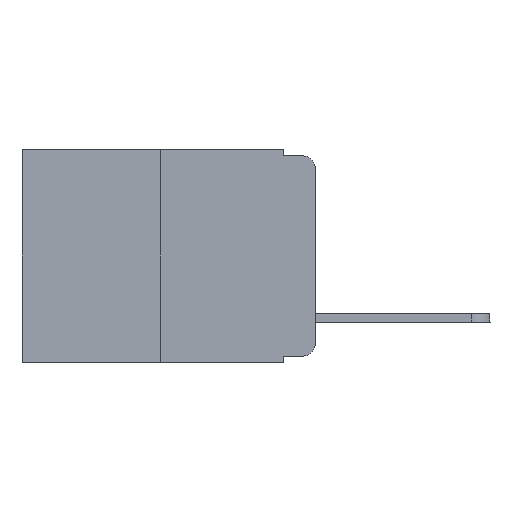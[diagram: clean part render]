
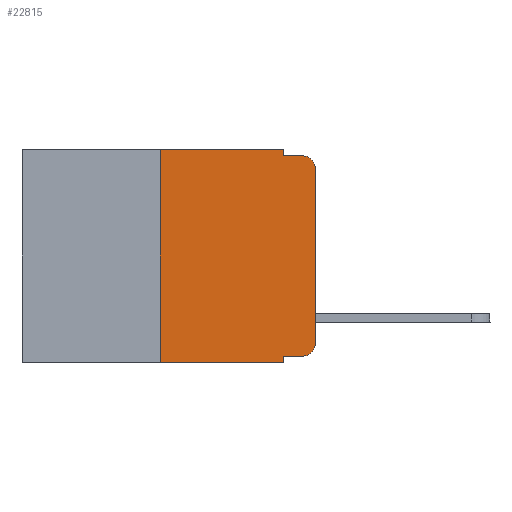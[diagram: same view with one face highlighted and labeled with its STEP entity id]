
A CAD part, left-side view. The second image highlights one B-rep face of the part: STEP entity #22815.
In plain terms, the highlighted planar face has unit normal (-1, 0, 0).
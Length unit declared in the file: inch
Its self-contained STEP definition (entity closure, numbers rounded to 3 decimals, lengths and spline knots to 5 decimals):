
#194 = VERTEX_POINT ( 'NONE', #18640 ) ;
#509 = AXIS2_PLACEMENT_3D ( 'NONE', #10040, #17757, #15505 ) ;
#854 = LINE ( 'NONE', #21071, #17240 ) ;
#1077 = VERTEX_POINT ( 'NONE', #19638 ) ;
#1090 = ORIENTED_EDGE ( 'NONE', *, *, #5804, .F. ) ;
#1209 = VERTEX_POINT ( 'NONE', #13346 ) ;
#1763 = VERTEX_POINT ( 'NONE', #2356 ) ;
#2220 = DIRECTION ( 'NONE',  ( 0., 0., 1. ) ) ;
#2356 = CARTESIAN_POINT ( 'NONE',  ( 0., 0.051, -0.01 ) ) ;
#3010 = VECTOR ( 'NONE', #23158, 39.37008 ) ;
#3176 = VERTEX_POINT ( 'NONE', #6206 ) ;
#3215 = CARTESIAN_POINT ( 'NONE',  ( 0., 0.051, -0.01 ) ) ;
#4160 = CIRCLE ( 'NONE', #19452, 0.02 ) ;
#4940 = VECTOR ( 'NONE', #9705, 39.37008 ) ;
#5382 = VERTEX_POINT ( 'NONE', #6452 ) ;
#5804 = EDGE_CURVE ( 'NONE', #1077, #10270, #8933, .T. ) ;
#5820 = LINE ( 'NONE', #3215, #4940 ) ;
#6116 = ORIENTED_EDGE ( 'NONE', *, *, #10657, .T. ) ;
#6206 = CARTESIAN_POINT ( 'NONE',  ( 0., 0., -0.03 ) ) ;
#6226 = CARTESIAN_POINT ( 'NONE',  ( 0., 0.02, -0.03 ) ) ;
#6452 = CARTESIAN_POINT ( 'NONE',  ( 0., 0.25, -0.343 ) ) ;
#6763 = ORIENTED_EDGE ( 'NONE', *, *, #11725, .T. ) ;
#6996 = ORIENTED_EDGE ( 'NONE', *, *, #19498, .F. ) ;
#7298 = CARTESIAN_POINT ( 'NONE',  ( 0., 0.051, 0. ) ) ;
#7810 = DIRECTION ( 'NONE',  ( 0., 0., -1. ) ) ;
#8051 = CARTESIAN_POINT ( 'NONE',  ( 0., 0.473, 0. ) ) ;
#8629 = ORIENTED_EDGE ( 'NONE', *, *, #8734, .T. ) ;
#8734 = EDGE_CURVE ( 'NONE', #194, #11779, #18633, .T. ) ;
#8880 = LINE ( 'NONE', #19145, #15117 ) ;
#8933 = LINE ( 'NONE', #7298, #20874 ) ;
#9314 = CARTESIAN_POINT ( 'NONE',  ( 0., 0., -0.313 ) ) ;
#9377 = ORIENTED_EDGE ( 'NONE', *, *, #12664, .T. ) ;
#9502 = CARTESIAN_POINT ( 'NONE',  ( 0., 0., 0. ) ) ;
#9517 = LINE ( 'NONE', #13839, #16633 ) ;
#9705 = DIRECTION ( 'NONE',  ( 0., -1., 0. ) ) ;
#9771 = CARTESIAN_POINT ( 'NONE',  ( 0., 0.051, -0.333 ) ) ;
#10040 = CARTESIAN_POINT ( 'NONE',  ( 0., 0.02, -0.313 ) ) ;
#10270 = VERTEX_POINT ( 'NONE', #10436 ) ;
#10436 = CARTESIAN_POINT ( 'NONE',  ( 0., 0.051, -0.343 ) ) ;
#10657 = EDGE_CURVE ( 'NONE', #1077, #194, #13467, .T. ) ;
#10731 = ORIENTED_EDGE ( 'NONE', *, *, #11717, .F. ) ;
#11422 = ORIENTED_EDGE ( 'NONE', *, *, #20151, .F. ) ;
#11717 = EDGE_CURVE ( 'NONE', #20678, #1763, #854, .T. ) ;
#11722 = DIRECTION ( 'NONE',  ( 0., 0., -1. ) ) ;
#11725 = EDGE_CURVE ( 'NONE', #11779, #3176, #18440, .T. ) ;
#11779 = VERTEX_POINT ( 'NONE', #9314 ) ;
#12202 = VECTOR ( 'NONE', #2220, 39.37008 ) ;
#12288 = ORIENTED_EDGE ( 'NONE', *, *, #24498, .T. ) ;
#12664 = EDGE_CURVE ( 'NONE', #5382, #10270, #9517, .T. ) ;
#13051 = ORIENTED_EDGE ( 'NONE', *, *, #19411, .F. ) ;
#13346 = CARTESIAN_POINT ( 'NONE',  ( 0., 0.02, -0.01 ) ) ;
#13467 = LINE ( 'NONE', #9771, #3010 ) ;
#13555 = DIRECTION ( 'NONE',  ( 1., 0., 0. ) ) ;
#13806 = PLANE ( 'NONE',  #21669 ) ;
#13839 = CARTESIAN_POINT ( 'NONE',  ( 0., 0.473, -0.343 ) ) ;
#14164 = VECTOR ( 'NONE', #20880, 39.37008 ) ;
#15117 = VECTOR ( 'NONE', #19065, 39.37008 ) ;
#15505 = DIRECTION ( 'NONE',  ( 0., 0., -1. ) ) ;
#15634 = DIRECTION ( 'NONE',  ( 0., 0., -1. ) ) ;
#15910 = DIRECTION ( 'NONE',  ( 0., -1., 0. ) ) ;
#16633 = VECTOR ( 'NONE', #15910, 39.37008 ) ;
#16689 = EDGE_LOOP ( 'NONE', ( #6763, #12288, #13051, #10731, #6996, #11422, #9377, #1090, #6116, #8629 ) ) ;
#17017 = CARTESIAN_POINT ( 'NONE',  ( 0., 0.473, 0. ) ) ;
#17240 = VECTOR ( 'NONE', #7810, 39.37008 ) ;
#17757 = DIRECTION ( 'NONE',  ( -1., 0., 0. ) ) ;
#18440 = LINE ( 'NONE', #9502, #12202 ) ;
#18633 = CIRCLE ( 'NONE', #509, 0.02 ) ;
#18640 = CARTESIAN_POINT ( 'NONE',  ( 0., 0.02, -0.333 ) ) ;
#18899 = LINE ( 'NONE', #17017, #14164 ) ;
#19065 = DIRECTION ( 'NONE',  ( 0., 0., 1. ) ) ;
#19145 = CARTESIAN_POINT ( 'NONE',  ( 0., 0.25, 0. ) ) ;
#19411 = EDGE_CURVE ( 'NONE', #1763, #1209, #5820, .T. ) ;
#19452 = AXIS2_PLACEMENT_3D ( 'NONE', #6226, #23375, #15634 ) ;
#19498 = EDGE_CURVE ( 'NONE', #21715, #20678, #18899, .T. ) ;
#19638 = CARTESIAN_POINT ( 'NONE',  ( 0., 0.051, -0.333 ) ) ;
#20151 = EDGE_CURVE ( 'NONE', #5382, #21715, #8880, .T. ) ;
#20460 = DIRECTION ( 'NONE',  ( 0., 0., -1. ) ) ;
#20657 = CARTESIAN_POINT ( 'NONE',  ( 0., 0.051, 0. ) ) ;
#20678 = VERTEX_POINT ( 'NONE', #20657 ) ;
#20874 = VECTOR ( 'NONE', #20460, 39.37008 ) ;
#20880 = DIRECTION ( 'NONE',  ( 0., -1., 0. ) ) ;
#21071 = CARTESIAN_POINT ( 'NONE',  ( 0., 0.051, 0. ) ) ;
#21669 = AXIS2_PLACEMENT_3D ( 'NONE', #8051, #13555, #11722 ) ;
#21715 = VERTEX_POINT ( 'NONE', #21763 ) ;
#21763 = CARTESIAN_POINT ( 'NONE',  ( 0., 0.25, 0. ) ) ;
#22747 = FACE_OUTER_BOUND ( 'NONE', #16689, .T. ) ;
#22815 = ADVANCED_FACE ( 'NONE', ( #22747 ), #13806, .F. ) ;
#23158 = DIRECTION ( 'NONE',  ( 0., -1., 0. ) ) ;
#23375 = DIRECTION ( 'NONE',  ( -1., 0., 0. ) ) ;
#24498 = EDGE_CURVE ( 'NONE', #3176, #1209, #4160, .T. ) ;
